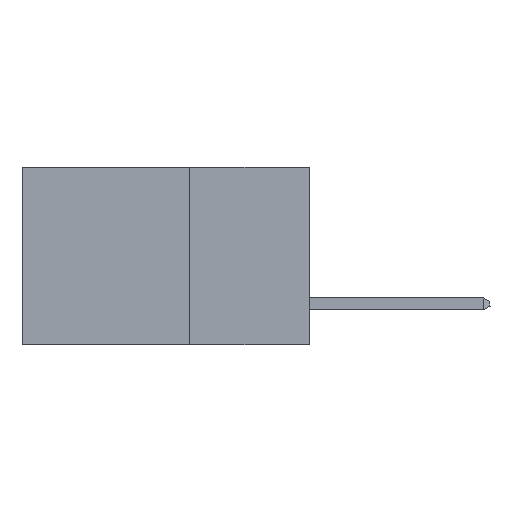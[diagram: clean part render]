
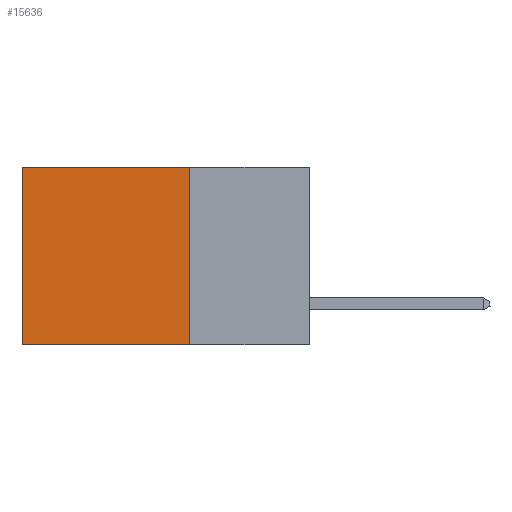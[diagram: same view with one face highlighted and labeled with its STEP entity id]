
A CAD part, left-side view. The second image highlights one B-rep face of the part: STEP entity #15636.
In plain terms, the highlighted planar face has unit normal (-1, 0, 0).
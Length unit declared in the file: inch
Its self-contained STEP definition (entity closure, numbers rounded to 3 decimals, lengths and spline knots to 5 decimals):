
#615 = CARTESIAN_POINT ( 'NONE',  ( 0.2875, 0.25, -0.37 ) ) ;
#1186 = CARTESIAN_POINT ( 'NONE',  ( 0.2875, 0.25, 0. ) ) ;
#2464 = EDGE_CURVE ( 'NONE', #20158, #22020, #5348, .T. ) ;
#3720 = VERTEX_POINT ( 'NONE', #615 ) ;
#3786 = ORIENTED_EDGE ( 'NONE', *, *, #2464, .T. ) ;
#3966 = FACE_OUTER_BOUND ( 'NONE', #7636, .T. ) ;
#3981 = PLANE ( 'NONE',  #18588 ) ;
#4260 = LINE ( 'NONE', #20909, #18654 ) ;
#5057 = VERTEX_POINT ( 'NONE', #9745 ) ;
#5348 = LINE ( 'NONE', #14873, #11376 ) ;
#7041 = ORIENTED_EDGE ( 'NONE', *, *, #21022, .F. ) ;
#7207 = DIRECTION ( 'NONE',  ( 0., 0., -1. ) ) ;
#7325 = DIRECTION ( 'NONE',  ( 1., 0., 0. ) ) ;
#7636 = EDGE_LOOP ( 'NONE', ( #3786, #7904, #7041, #12193 ) ) ;
#7904 = ORIENTED_EDGE ( 'NONE', *, *, #16090, .F. ) ;
#9373 = CARTESIAN_POINT ( 'NONE',  ( 0.2875, 0.6, -0.37 ) ) ;
#9745 = CARTESIAN_POINT ( 'NONE',  ( 0.2875, 0.25, 0. ) ) ;
#11376 = VECTOR ( 'NONE', #13054, 39.37008 ) ;
#11617 = VECTOR ( 'NONE', #7207, 39.37008 ) ;
#12193 = ORIENTED_EDGE ( 'NONE', *, *, #21749, .T. ) ;
#12623 = LINE ( 'NONE', #15089, #21264 ) ;
#13054 = DIRECTION ( 'NONE',  ( 0., 0., -1. ) ) ;
#14873 = CARTESIAN_POINT ( 'NONE',  ( 0.2875, 0.6, 0. ) ) ;
#15089 = CARTESIAN_POINT ( 'NONE',  ( 0.2875, 0.25, -0.37 ) ) ;
#15636 = ADVANCED_FACE ( 'NONE', ( #3966 ), #3981, .F. ) ;
#15703 = DIRECTION ( 'NONE',  ( 0., 1., 0. ) ) ;
#15813 = CARTESIAN_POINT ( 'NONE',  ( 0.2875, 0.6, 0. ) ) ;
#16090 = EDGE_CURVE ( 'NONE', #3720, #22020, #12623, .T. ) ;
#17846 = DIRECTION ( 'NONE',  ( 0., 0., -1. ) ) ;
#18513 = DIRECTION ( 'NONE',  ( 0., 1., 0. ) ) ;
#18588 = AXIS2_PLACEMENT_3D ( 'NONE', #19426, #7325, #17846 ) ;
#18654 = VECTOR ( 'NONE', #15703, 39.37008 ) ;
#19426 = CARTESIAN_POINT ( 'NONE',  ( 0.2875, 0.25, 0. ) ) ;
#20158 = VERTEX_POINT ( 'NONE', #15813 ) ;
#20909 = CARTESIAN_POINT ( 'NONE',  ( 0.2875, 0.25, 0. ) ) ;
#21022 = EDGE_CURVE ( 'NONE', #5057, #3720, #21028, .T. ) ;
#21028 = LINE ( 'NONE', #1186, #11617 ) ;
#21264 = VECTOR ( 'NONE', #18513, 39.37008 ) ;
#21749 = EDGE_CURVE ( 'NONE', #5057, #20158, #4260, .T. ) ;
#22020 = VERTEX_POINT ( 'NONE', #9373 ) ;
